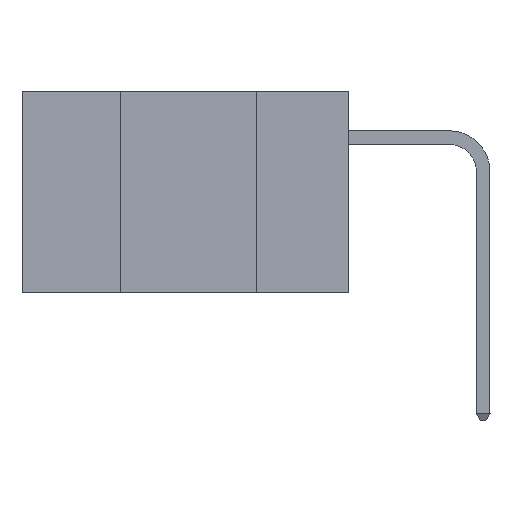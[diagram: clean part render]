
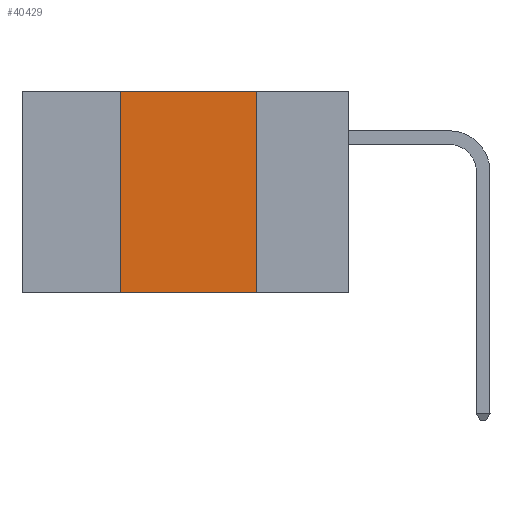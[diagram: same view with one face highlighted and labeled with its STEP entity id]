
A CAD part, left-side view. The second image highlights one B-rep face of the part: STEP entity #40429.
In plain terms, the highlighted planar face has unit normal (-1, 0, 0).
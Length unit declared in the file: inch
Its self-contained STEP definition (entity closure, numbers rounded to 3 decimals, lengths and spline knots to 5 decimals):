
#455 = CARTESIAN_POINT ( 'NONE',  ( 0., 0.6, -0.37 ) ) ;
#747 = CARTESIAN_POINT ( 'NONE',  ( 0., 0.6, 0. ) ) ;
#1022 = ORIENTED_EDGE ( 'NONE', *, *, #19839, .F. ) ;
#2475 = DIRECTION ( 'NONE',  ( 0., 0., 1. ) ) ;
#2841 = ORIENTED_EDGE ( 'NONE', *, *, #32482, .T. ) ;
#3999 = EDGE_CURVE ( 'NONE', #15624, #32783, #15805, .T. ) ;
#6990 = CARTESIAN_POINT ( 'NONE',  ( 0., 0.17, -0.37 ) ) ;
#8203 = CARTESIAN_POINT ( 'NONE',  ( 0., 0.6, 0. ) ) ;
#9458 = VERTEX_POINT ( 'NONE', #32649 ) ;
#9813 = VECTOR ( 'NONE', #19780, 39.37008 ) ;
#12218 = CARTESIAN_POINT ( 'NONE',  ( 0., 0.42, 0. ) ) ;
#12930 = FACE_OUTER_BOUND ( 'NONE', #38804, .T. ) ;
#14878 = CARTESIAN_POINT ( 'NONE',  ( 0., 0.42, 0. ) ) ;
#15454 = EDGE_CURVE ( 'NONE', #9458, #21675, #34000, .T. ) ;
#15510 = ORIENTED_EDGE ( 'NONE', *, *, #3999, .F. ) ;
#15624 = VERTEX_POINT ( 'NONE', #38381 ) ;
#15805 = LINE ( 'NONE', #25070, #31399 ) ;
#19244 = DIRECTION ( 'NONE',  ( 0., 0., -1. ) ) ;
#19780 = DIRECTION ( 'NONE',  ( 0., -1., 0. ) ) ;
#19839 = EDGE_CURVE ( 'NONE', #21675, #15624, #27329, .T. ) ;
#19870 = PLANE ( 'NONE',  #25618 ) ;
#20080 = DIRECTION ( 'NONE',  ( 1., 0., 0. ) ) ;
#21675 = VERTEX_POINT ( 'NONE', #12218 ) ;
#21801 = VECTOR ( 'NONE', #2475, 39.37008 ) ;
#24178 = DIRECTION ( 'NONE',  ( 0., -1., 0. ) ) ;
#25070 = CARTESIAN_POINT ( 'NONE',  ( 0., 0.17, 0. ) ) ;
#25618 = AXIS2_PLACEMENT_3D ( 'NONE', #747, #20080, #19244 ) ;
#27329 = LINE ( 'NONE', #8203, #32094 ) ;
#29225 = LINE ( 'NONE', #455, #9813 ) ;
#31397 = ORIENTED_EDGE ( 'NONE', *, *, #15454, .F. ) ;
#31399 = VECTOR ( 'NONE', #31775, 39.37008 ) ;
#31775 = DIRECTION ( 'NONE',  ( 0., 0., -1. ) ) ;
#32094 = VECTOR ( 'NONE', #24178, 39.37008 ) ;
#32482 = EDGE_CURVE ( 'NONE', #9458, #32783, #29225, .T. ) ;
#32649 = CARTESIAN_POINT ( 'NONE',  ( 0., 0.42, -0.37 ) ) ;
#32783 = VERTEX_POINT ( 'NONE', #6990 ) ;
#34000 = LINE ( 'NONE', #14878, #21801 ) ;
#38381 = CARTESIAN_POINT ( 'NONE',  ( 0., 0.17, 0. ) ) ;
#38804 = EDGE_LOOP ( 'NONE', ( #15510, #1022, #31397, #2841 ) ) ;
#40429 = ADVANCED_FACE ( 'NONE', ( #12930 ), #19870, .F. ) ;
